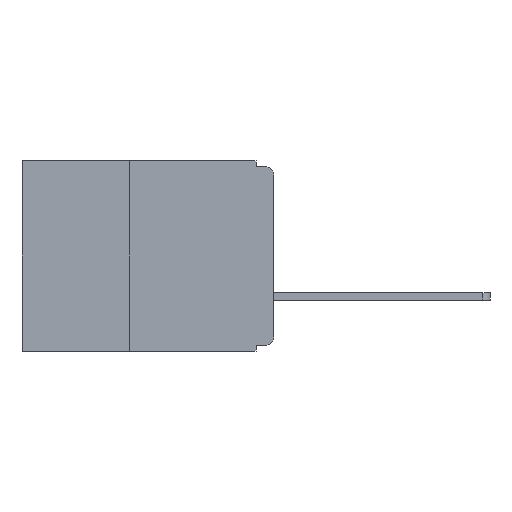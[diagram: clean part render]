
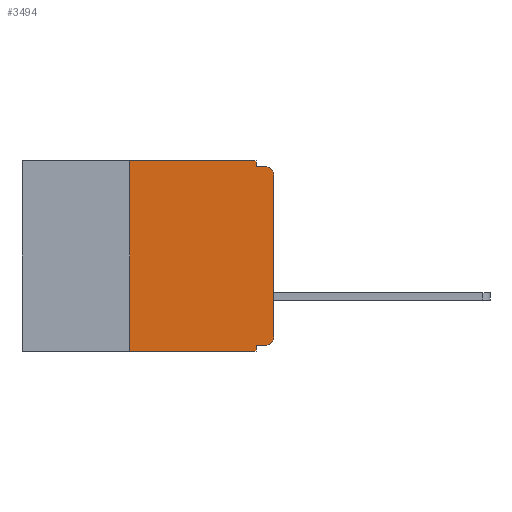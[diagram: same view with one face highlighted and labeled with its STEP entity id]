
A CAD part, left-side view. The second image highlights one B-rep face of the part: STEP entity #3494.
In plain terms, the highlighted planar face has unit normal (-1, 0, 0).
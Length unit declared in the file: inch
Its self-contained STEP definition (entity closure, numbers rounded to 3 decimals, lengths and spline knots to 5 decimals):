
#99 = AXIS2_PLACEMENT_3D ( 'NONE', #10791, #4149, #11814 ) ;
#158 = VECTOR ( 'NONE', #8118, 39.37008 ) ;
#446 = CARTESIAN_POINT ( 'NONE',  ( 0., 0.25, 0. ) ) ;
#862 = EDGE_LOOP ( 'NONE', ( #6596, #9535, #9868, #4218, #7322, #10188, #1381, #7659, #1801, #4971 ) ) ;
#1305 = EDGE_CURVE ( 'NONE', #4827, #2293, #7362, .T. ) ;
#1381 = ORIENTED_EDGE ( 'NONE', *, *, #2017, .T. ) ;
#1709 = DIRECTION ( 'NONE',  ( 0., 0., -1. ) ) ;
#1753 = VERTEX_POINT ( 'NONE', #5279 ) ;
#1801 = ORIENTED_EDGE ( 'NONE', *, *, #1305, .F. ) ;
#1842 = VERTEX_POINT ( 'NONE', #446 ) ;
#1855 = VERTEX_POINT ( 'NONE', #5941 ) ;
#1901 = VECTOR ( 'NONE', #3642, 39.37008 ) ;
#1905 = EDGE_CURVE ( 'NONE', #1855, #6591, #5360, .T. ) ;
#1937 = CARTESIAN_POINT ( 'NONE',  ( 0., 0., -0.305 ) ) ;
#1977 = EDGE_CURVE ( 'NONE', #7792, #1842, #12233, .T. ) ;
#2017 = EDGE_CURVE ( 'NONE', #7792, #8171, #3161, .T. ) ;
#2036 = VERTEX_POINT ( 'NONE', #6601 ) ;
#2124 = EDGE_CURVE ( 'NONE', #2293, #8171, #4792, .T. ) ;
#2133 = FACE_OUTER_BOUND ( 'NONE', #862, .T. ) ;
#2293 = VERTEX_POINT ( 'NONE', #12988 ) ;
#2424 = CARTESIAN_POINT ( 'NONE',  ( 0., 0., -0.01 ) ) ;
#2739 = LINE ( 'NONE', #4691, #11250 ) ;
#2938 = CARTESIAN_POINT ( 'NONE',  ( 0., 0.437, 0. ) ) ;
#3161 = LINE ( 'NONE', #9411, #11627 ) ;
#3226 = AXIS2_PLACEMENT_3D ( 'NONE', #14089, #14013, #14001 ) ;
#3245 = DIRECTION ( 'NONE',  ( 0., 1., 0. ) ) ;
#3343 = CARTESIAN_POINT ( 'NONE',  ( 0., 0.031, -0.01 ) ) ;
#3494 = ADVANCED_FACE ( 'NONE', ( #2133 ), #5217, .F. ) ;
#3550 = DIRECTION ( 'NONE',  ( 0., 0., -1. ) ) ;
#3563 = DIRECTION ( 'NONE',  ( 1., 0., 0. ) ) ;
#3642 = DIRECTION ( 'NONE',  ( 0., -1., 0. ) ) ;
#3679 = CARTESIAN_POINT ( 'NONE',  ( 0., 0.437, 0. ) ) ;
#3872 = CARTESIAN_POINT ( 'NONE',  ( 0., 0.031, 0. ) ) ;
#4149 = DIRECTION ( 'NONE',  ( -1., 0., 0. ) ) ;
#4218 = ORIENTED_EDGE ( 'NONE', *, *, #1905, .F. ) ;
#4252 = VECTOR ( 'NONE', #3245, 39.37008 ) ;
#4691 = CARTESIAN_POINT ( 'NONE',  ( 0., 0., 0. ) ) ;
#4792 = LINE ( 'NONE', #7043, #12689 ) ;
#4827 = VERTEX_POINT ( 'NONE', #6355 ) ;
#4971 = ORIENTED_EDGE ( 'NONE', *, *, #5142, .T. ) ;
#4983 = VECTOR ( 'NONE', #7510, 39.37008 ) ;
#5142 = EDGE_CURVE ( 'NONE', #4827, #13153, #6711, .T. ) ;
#5217 = PLANE ( 'NONE',  #5734 ) ;
#5279 = CARTESIAN_POINT ( 'NONE',  ( 0., 0.015, -0.01 ) ) ;
#5360 = LINE ( 'NONE', #3872, #4983 ) ;
#5664 = CIRCLE ( 'NONE', #99, 0.015 ) ;
#5734 = AXIS2_PLACEMENT_3D ( 'NONE', #3679, #3563, #3550 ) ;
#5941 = CARTESIAN_POINT ( 'NONE',  ( 0., 0.031, 0. ) ) ;
#6275 = DIRECTION ( 'NONE',  ( 0., -1., 0. ) ) ;
#6355 = CARTESIAN_POINT ( 'NONE',  ( 0., 0.015, -0.32 ) ) ;
#6491 = LINE ( 'NONE', #2938, #11528 ) ;
#6591 = VERTEX_POINT ( 'NONE', #3343 ) ;
#6596 = ORIENTED_EDGE ( 'NONE', *, *, #12681, .T. ) ;
#6601 = CARTESIAN_POINT ( 'NONE',  ( 0., 0., -0.025 ) ) ;
#6711 = CIRCLE ( 'NONE', #3226, 0.015 ) ;
#7043 = CARTESIAN_POINT ( 'NONE',  ( 0., 0.031, -0.33 ) ) ;
#7251 = EDGE_CURVE ( 'NONE', #1842, #1855, #6491, .T. ) ;
#7322 = ORIENTED_EDGE ( 'NONE', *, *, #7251, .F. ) ;
#7362 = LINE ( 'NONE', #10544, #4252 ) ;
#7508 = CARTESIAN_POINT ( 'NONE',  ( 0., 0.25, -0.33 ) ) ;
#7510 = DIRECTION ( 'NONE',  ( 0., 0., -1. ) ) ;
#7659 = ORIENTED_EDGE ( 'NONE', *, *, #2124, .F. ) ;
#7792 = VERTEX_POINT ( 'NONE', #7508 ) ;
#8118 = DIRECTION ( 'NONE',  ( 0., 0., 1. ) ) ;
#8171 = VERTEX_POINT ( 'NONE', #11234 ) ;
#9411 = CARTESIAN_POINT ( 'NONE',  ( 0., 0.437, -0.33 ) ) ;
#9483 = CARTESIAN_POINT ( 'NONE',  ( 0., 0.25, -0.33 ) ) ;
#9535 = ORIENTED_EDGE ( 'NONE', *, *, #12026, .T. ) ;
#9868 = ORIENTED_EDGE ( 'NONE', *, *, #13990, .F. ) ;
#10188 = ORIENTED_EDGE ( 'NONE', *, *, #1977, .F. ) ;
#10544 = CARTESIAN_POINT ( 'NONE',  ( 0., 0., -0.32 ) ) ;
#10791 = CARTESIAN_POINT ( 'NONE',  ( 0., 0.015, -0.025 ) ) ;
#10895 = LINE ( 'NONE', #2424, #1901 ) ;
#11234 = CARTESIAN_POINT ( 'NONE',  ( 0., 0.031, -0.33 ) ) ;
#11250 = VECTOR ( 'NONE', #14182, 39.37008 ) ;
#11528 = VECTOR ( 'NONE', #12728, 39.37008 ) ;
#11627 = VECTOR ( 'NONE', #6275, 39.37008 ) ;
#11814 = DIRECTION ( 'NONE',  ( 0., 0., -1. ) ) ;
#12026 = EDGE_CURVE ( 'NONE', #2036, #1753, #5664, .T. ) ;
#12233 = LINE ( 'NONE', #9483, #158 ) ;
#12681 = EDGE_CURVE ( 'NONE', #13153, #2036, #2739, .T. ) ;
#12689 = VECTOR ( 'NONE', #1709, 39.37008 ) ;
#12728 = DIRECTION ( 'NONE',  ( 0., -1., 0. ) ) ;
#12988 = CARTESIAN_POINT ( 'NONE',  ( 0., 0.031, -0.32 ) ) ;
#13153 = VERTEX_POINT ( 'NONE', #1937 ) ;
#13990 = EDGE_CURVE ( 'NONE', #6591, #1753, #10895, .T. ) ;
#14001 = DIRECTION ( 'NONE',  ( 0., 0., -1. ) ) ;
#14013 = DIRECTION ( 'NONE',  ( -1., 0., 0. ) ) ;
#14089 = CARTESIAN_POINT ( 'NONE',  ( 0., 0.015, -0.305 ) ) ;
#14182 = DIRECTION ( 'NONE',  ( 0., 0., 1. ) ) ;
